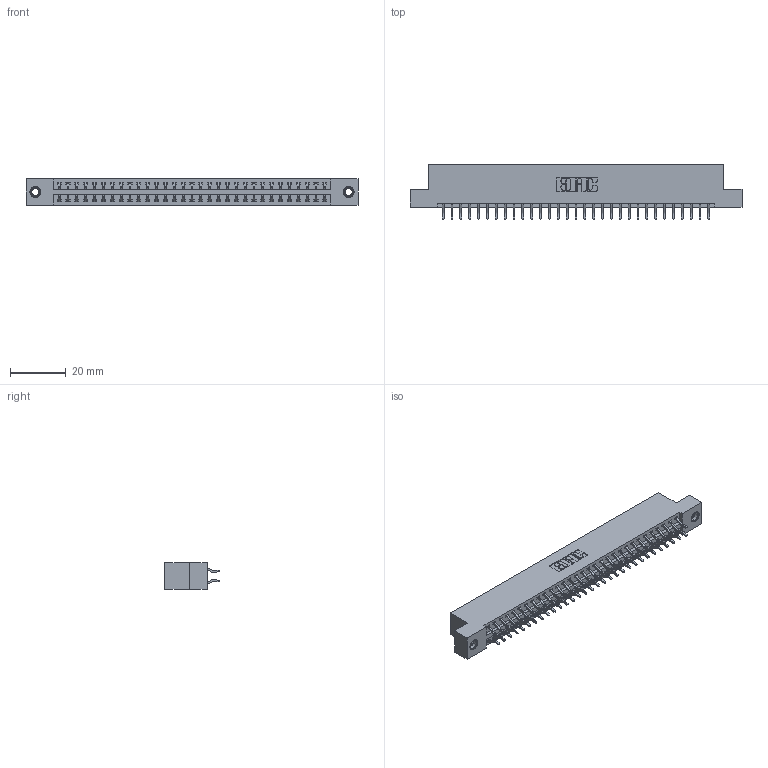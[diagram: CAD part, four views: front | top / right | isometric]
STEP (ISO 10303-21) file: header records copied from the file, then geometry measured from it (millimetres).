
FILE_DESCRIPTION (( 'STEP AP203' ), '1' );
FILE_NAME ('346-062-556-207.STEP', '2018-08-28T07:47:42', ( '' ), ( '' ), 'SwSTEP 2.0', 'SolidWorks 2016', '' );
FILE_SCHEMA (( 'CONFIG_CONTROL_DESIGN' ));
Length unit declared in the file: inch
Products named in the file (4): 345-250-001_345-250-005-103; 346-062-556-207; 346 Part_Flush Mounting Lugs - 0.156 Dia-TI; 345-292-001_556 Tail
Assembly tree (65 placements, depth 2):
  346-062-556-207
    346 Part_Flush Mounting Lugs - 0.156 Dia-TI
    345-292-001_556 Tail  x62
    345-250-001_345-250-005-103  x2
Bounding box: 119 x 19.57 x 9.4 mm (x, y, z)
Volume: 11502.5 mm3; surface area: 15614.2 mm2
Topology: 65 solids, 65 shells, 3778 faces, 11191 edges, 7370 vertices
Faces by surface type: plane 2526, cylinder 1236, cone 12, torus 4
Entity records: 23118 total; most frequent: CARTESIAN_POINT 3823, ORIENTED_EDGE 3738, DIRECTION 3435, EDGE_CURVE 1869, VECTOR 1585, LINE 1585, VERTEX_POINT 1240, AXIS2_PLACEMENT_3D 925
